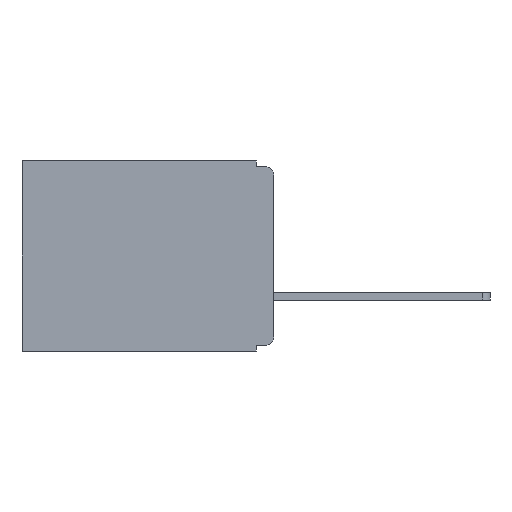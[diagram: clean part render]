
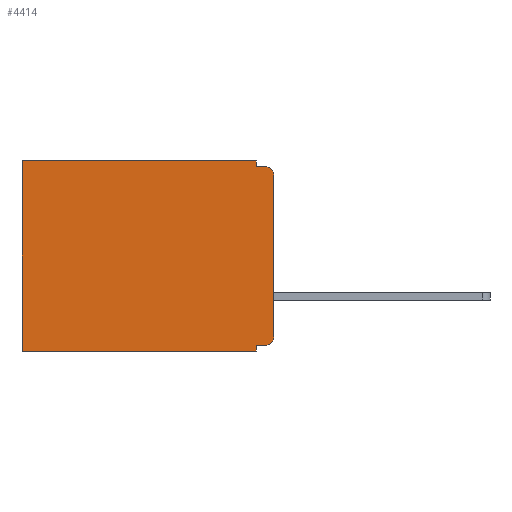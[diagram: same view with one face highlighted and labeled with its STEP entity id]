
A CAD part, left-side view. The second image highlights one B-rep face of the part: STEP entity #4414.
In plain terms, the highlighted planar face has unit normal (-1, 0, 0).
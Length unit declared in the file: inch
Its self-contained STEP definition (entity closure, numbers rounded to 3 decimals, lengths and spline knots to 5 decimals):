
#50 = VERTEX_POINT ( 'NONE', #7473 ) ;
#125 = CARTESIAN_POINT ( 'NONE',  ( 0.3, 0.031, -0.01 ) ) ;
#273 = AXIS2_PLACEMENT_3D ( 'NONE', #2321, #2297, #2294 ) ;
#295 = LINE ( 'NONE', #10455, #3353 ) ;
#438 = EDGE_CURVE ( 'NONE', #5217, #6908, #10274, .T. ) ;
#755 = CARTESIAN_POINT ( 'NONE',  ( 0.3, 0.437, 0. ) ) ;
#965 = VERTEX_POINT ( 'NONE', #10030 ) ;
#1355 = VERTEX_POINT ( 'NONE', #6633 ) ;
#1392 = DIRECTION ( 'NONE',  ( 0., 0., -1. ) ) ;
#1447 = AXIS2_PLACEMENT_3D ( 'NONE', #2473, #2445, #2441 ) ;
#1789 = CARTESIAN_POINT ( 'NONE',  ( 0.3, 0.031, -0.33 ) ) ;
#1819 = VERTEX_POINT ( 'NONE', #1945 ) ;
#1834 = LINE ( 'NONE', #5321, #1892 ) ;
#1892 = VECTOR ( 'NONE', #5475, 39.37008 ) ;
#1945 = CARTESIAN_POINT ( 'NONE',  ( 0.3, 0.031, -0.32 ) ) ;
#2126 = VECTOR ( 'NONE', #4645, 39.37008 ) ;
#2294 = DIRECTION ( 'NONE',  ( 0., 0., -1. ) ) ;
#2297 = DIRECTION ( 'NONE',  ( -1., 0., 0. ) ) ;
#2321 = CARTESIAN_POINT ( 'NONE',  ( 0.3, 0.015, -0.305 ) ) ;
#2441 = DIRECTION ( 'NONE',  ( 0., 0., -1. ) ) ;
#2445 = DIRECTION ( 'NONE',  ( -1., 0., 0. ) ) ;
#2473 = CARTESIAN_POINT ( 'NONE',  ( 0.3, 0.015, -0.025 ) ) ;
#2505 = DIRECTION ( 'NONE',  ( 0., 1., 0. ) ) ;
#2589 = DIRECTION ( 'NONE',  ( 1., 0., 0. ) ) ;
#3157 = DIRECTION ( 'NONE',  ( 0., 1., 0. ) ) ;
#3179 = CARTESIAN_POINT ( 'NONE',  ( 0.3, 0., -0.32 ) ) ;
#3353 = VECTOR ( 'NONE', #6567, 39.37008 ) ;
#3650 = VERTEX_POINT ( 'NONE', #1789 ) ;
#3686 = DIRECTION ( 'NONE',  ( 0., 0., -1. ) ) ;
#3961 = LINE ( 'NONE', #4728, #2126 ) ;
#3984 = EDGE_CURVE ( 'NONE', #6908, #4195, #295, .T. ) ;
#4195 = VERTEX_POINT ( 'NONE', #6914 ) ;
#4233 = CARTESIAN_POINT ( 'NONE',  ( 0.3, 0., -0.33 ) ) ;
#4268 = CARTESIAN_POINT ( 'NONE',  ( 0.3, 0.031, 0. ) ) ;
#4279 = DIRECTION ( 'NONE',  ( 0., 1., 0. ) ) ;
#4414 = ADVANCED_FACE ( 'NONE', ( #7021 ), #6177, .F. ) ;
#4645 = DIRECTION ( 'NONE',  ( 0., -1., 0. ) ) ;
#4728 = CARTESIAN_POINT ( 'NONE',  ( 0.3, 0., -0.01 ) ) ;
#4795 = VERTEX_POINT ( 'NONE', #125 ) ;
#5217 = VERTEX_POINT ( 'NONE', #4268 ) ;
#5321 = CARTESIAN_POINT ( 'NONE',  ( 0.3, 0., -0.33 ) ) ;
#5475 = DIRECTION ( 'NONE',  ( 0., 0., -1. ) ) ;
#5480 = ORIENTED_EDGE ( 'NONE', *, *, #6602, .T. ) ;
#5806 = ORIENTED_EDGE ( 'NONE', *, *, #6477, .F. ) ;
#5876 = ORIENTED_EDGE ( 'NONE', *, *, #7653, .F. ) ;
#5877 = CARTESIAN_POINT ( 'NONE',  ( 0.3, 0., 0. ) ) ;
#6094 = VECTOR ( 'NONE', #3686, 39.37008 ) ;
#6177 = PLANE ( 'NONE',  #6258 ) ;
#6258 = AXIS2_PLACEMENT_3D ( 'NONE', #6418, #2589, #1392 ) ;
#6268 = EDGE_CURVE ( 'NONE', #1355, #7360, #1834, .T. ) ;
#6356 = EDGE_CURVE ( 'NONE', #4795, #50, #3961, .T. ) ;
#6418 = CARTESIAN_POINT ( 'NONE',  ( 0.3, 0., -0.33 ) ) ;
#6477 = EDGE_CURVE ( 'NONE', #965, #1819, #10080, .T. ) ;
#6567 = DIRECTION ( 'NONE',  ( 0., 0., -1. ) ) ;
#6574 = EDGE_CURVE ( 'NONE', #1355, #50, #9772, .T. ) ;
#6602 = EDGE_CURVE ( 'NONE', #965, #7360, #9763, .T. ) ;
#6633 = CARTESIAN_POINT ( 'NONE',  ( 0.3, 0., -0.025 ) ) ;
#6856 = DIRECTION ( 'NONE',  ( 0., 0., -1. ) ) ;
#6877 = LINE ( 'NONE', #7296, #6094 ) ;
#6908 = VERTEX_POINT ( 'NONE', #755 ) ;
#6914 = CARTESIAN_POINT ( 'NONE',  ( 0.3, 0.437, -0.33 ) ) ;
#7021 = FACE_OUTER_BOUND ( 'NONE', #8675, .T. ) ;
#7058 = VECTOR ( 'NONE', #4279, 39.37008 ) ;
#7171 = VECTOR ( 'NONE', #6856, 39.37008 ) ;
#7296 = CARTESIAN_POINT ( 'NONE',  ( 0.3, 0.031, -0.33 ) ) ;
#7360 = VERTEX_POINT ( 'NONE', #7682 ) ;
#7473 = CARTESIAN_POINT ( 'NONE',  ( 0.3, 0.015, -0.01 ) ) ;
#7490 = EDGE_CURVE ( 'NONE', #3650, #4195, #10538, .T. ) ;
#7639 = EDGE_CURVE ( 'NONE', #5217, #4795, #8531, .T. ) ;
#7653 = EDGE_CURVE ( 'NONE', #1819, #3650, #6877, .T. ) ;
#7682 = CARTESIAN_POINT ( 'NONE',  ( 0.3, 0., -0.305 ) ) ;
#8531 = LINE ( 'NONE', #10512, #7171 ) ;
#8675 = EDGE_LOOP ( 'NONE', ( #9798, #9883, #9860, #10195, #9969, #10142, #9922, #5876, #5806, #5480 ) ) ;
#9763 = CIRCLE ( 'NONE', #273, 0.015 ) ;
#9772 = CIRCLE ( 'NONE', #1447, 0.015 ) ;
#9798 = ORIENTED_EDGE ( 'NONE', *, *, #6268, .F. ) ;
#9860 = ORIENTED_EDGE ( 'NONE', *, *, #6356, .F. ) ;
#9883 = ORIENTED_EDGE ( 'NONE', *, *, #6574, .T. ) ;
#9922 = ORIENTED_EDGE ( 'NONE', *, *, #7490, .F. ) ;
#9969 = ORIENTED_EDGE ( 'NONE', *, *, #438, .T. ) ;
#10030 = CARTESIAN_POINT ( 'NONE',  ( 0.3, 0.015, -0.32 ) ) ;
#10080 = LINE ( 'NONE', #3179, #10090 ) ;
#10090 = VECTOR ( 'NONE', #3157, 39.37008 ) ;
#10142 = ORIENTED_EDGE ( 'NONE', *, *, #3984, .T. ) ;
#10195 = ORIENTED_EDGE ( 'NONE', *, *, #7639, .F. ) ;
#10234 = VECTOR ( 'NONE', #2505, 39.37008 ) ;
#10274 = LINE ( 'NONE', #5877, #10234 ) ;
#10455 = CARTESIAN_POINT ( 'NONE',  ( 0.3, 0.437, -0.33 ) ) ;
#10512 = CARTESIAN_POINT ( 'NONE',  ( 0.3, 0.031, 0. ) ) ;
#10538 = LINE ( 'NONE', #4233, #7058 ) ;
